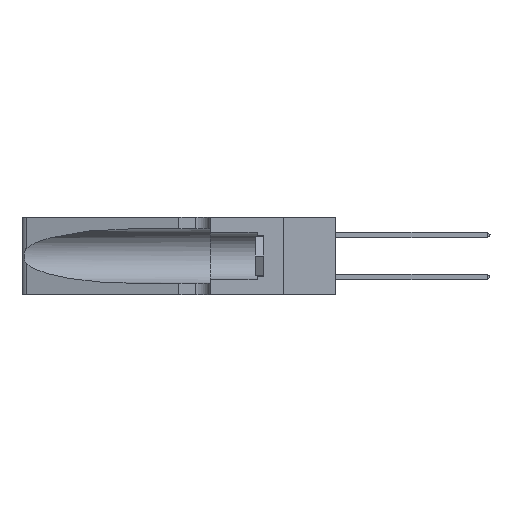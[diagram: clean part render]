
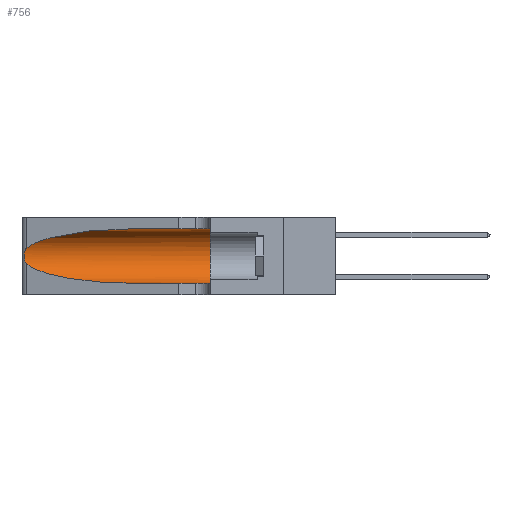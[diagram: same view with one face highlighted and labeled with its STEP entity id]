
A CAD part, left-side view. The second image highlights one B-rep face of the part: STEP entity #756.
In plain terms, the highlighted cylindrical face has radius 3.308 mm (diameter 6.617 mm), a partial arc.
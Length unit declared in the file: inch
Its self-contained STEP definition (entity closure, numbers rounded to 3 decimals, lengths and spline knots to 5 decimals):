
#478 = DIRECTION ( 'NONE',  ( 0., 1., 0. ) ) ;
#519 = CARTESIAN_POINT ( 'NONE',  ( 0.18966, 0.96281, 0.05475 ) ) ;
#756 = ADVANCED_FACE ( 'NONE', ( #10962 ), #19780, .F. ) ;
#801 = CARTESIAN_POINT ( 'NONE',  ( 0.1305, 0.35, 0.05475 ) ) ;
#1711 = CARTESIAN_POINT ( 'NONE',  ( 0.25639, 1.23186, 0.15144 ) ) ;
#2062 = CARTESIAN_POINT ( 'NONE',  ( 0.1305, 0.35, 0.31525 ) ) ;
#2937 = CARTESIAN_POINT ( 'NONE',  ( 0.25487, 1.22718, 0.22369 ) ) ;
#3628 = DIRECTION ( 'NONE',  ( 0., -1., 0. ) ) ;
#3702 = CARTESIAN_POINT ( 'NONE',  ( 0.25487, 1.22718, 0.14631 ) ) ;
#3805 = VECTOR ( 'NONE', #5480, 39.37008 ) ;
#3994 = VERTEX_POINT ( 'NONE', #6387 ) ;
#4312 = VERTEX_POINT ( 'NONE', #22398 ) ;
#4530 = VERTEX_POINT ( 'NONE', #24722 ) ;
#4669 = ORIENTED_EDGE ( 'NONE', *, *, #15088, .F. ) ;
#5480 = DIRECTION ( 'NONE',  ( 0., -1., 0. ) ) ;
#5661 = CARTESIAN_POINT ( 'NONE',  ( 0.25639, 1.23184, 0.21858 ) ) ;
#5757 =( BOUNDED_CURVE ( )  B_SPLINE_CURVE ( 3, ( #23375, #21598, #519, #14153 ),
 .UNSPECIFIED., .F., .F. ) 
 B_SPLINE_CURVE_WITH_KNOTS ( ( 4, 4 ),
 ( 3.44316, 4.71239 ),
 .UNSPECIFIED. ) 
 CURVE ( )  GEOMETRIC_REPRESENTATION_ITEM ( )  RATIONAL_B_SPLINE_CURVE ( ( 1., 0.87, 0.87, 1. ) ) 
 REPRESENTATION_ITEM ( '' )  );
#6387 = CARTESIAN_POINT ( 'NONE',  ( 0.1305, 0.72297, 0.31525 ) ) ;
#7619 = CARTESIAN_POINT ( 'NONE',  ( 0.25854, 1.2359, 0.20912 ) ) ;
#7921 = EDGE_CURVE ( 'NONE', #3994, #4530, #21419, .T. ) ;
#8882 = ORIENTED_EDGE ( 'NONE', *, *, #11031, .T. ) ;
#9578 = CARTESIAN_POINT ( 'NONE',  ( 0.26075, 1.23896, 0.19203 ) ) ;
#10030 = B_SPLINE_CURVE_WITH_KNOTS ( 'NONE', 3,
 ( #13295, #15187, #5661, #18964, #7619, #20837, #9578, #22679, #11482, #24537, #13374, #1711, #15270, #3702 ),
 .UNSPECIFIED., .F., .F.,
 ( 4, 2, 2, 2, 2, 2, 4 ),
 ( 0., 0.00027, 0.00053, 0.00107, 0.0016, 0.00187, 0.00214 ),
 .UNSPECIFIED. ) ;
#10962 = FACE_OUTER_BOUND ( 'NONE', #17174, .T. ) ;
#11031 = EDGE_CURVE ( 'NONE', #4530, #4312, #10030, .T. ) ;
#11482 = CARTESIAN_POINT ( 'NONE',  ( 0.26017, 1.23833, 0.17102 ) ) ;
#11982 = EDGE_CURVE ( 'NONE', #4312, #24225, #5757, .T. ) ;
#12139 = CARTESIAN_POINT ( 'NONE',  ( 0.1305, 1.61858, 0.185 ) ) ;
#12218 = CARTESIAN_POINT ( 'NONE',  ( 0.1305, 0.35, 0.185 ) ) ;
#12473 = ORIENTED_EDGE ( 'NONE', *, *, #11982, .T. ) ;
#12958 = DIRECTION ( 'NONE',  ( 0., -1., 0. ) ) ;
#13095 = VERTEX_POINT ( 'NONE', #2062 ) ;
#13295 = CARTESIAN_POINT ( 'NONE',  ( 0.25487, 1.22718, 0.22369 ) ) ;
#13374 = CARTESIAN_POINT ( 'NONE',  ( 0.25789, 1.23486, 0.15765 ) ) ;
#13762 = DIRECTION ( 'NONE',  ( 0., 0., -1. ) ) ;
#14127 = DIRECTION ( 'NONE',  ( 0., 0., 1. ) ) ;
#14153 = CARTESIAN_POINT ( 'NONE',  ( 0.1305, 0.72297, 0.05475 ) ) ;
#14269 = AXIS2_PLACEMENT_3D ( 'NONE', #12139, #12958, #13762 ) ;
#14525 = CARTESIAN_POINT ( 'NONE',  ( 0.2373, 1.15595, 0.28018 ) ) ;
#14857 = CARTESIAN_POINT ( 'NONE',  ( 0.1305, 0.72297, 0.05475 ) ) ;
#15036 = CARTESIAN_POINT ( 'NONE',  ( 0.1305, 1.61858, 0.31525 ) ) ;
#15088 = EDGE_CURVE ( 'NONE', #13095, #22888, #17392, .T. ) ;
#15187 = CARTESIAN_POINT ( 'NONE',  ( 0.25555, 1.22994, 0.2215 ) ) ;
#15270 = CARTESIAN_POINT ( 'NONE',  ( 0.25555, 1.22993, 0.14849 ) ) ;
#15970 = EDGE_CURVE ( 'NONE', #3994, #13095, #18520, .T. ) ;
#16364 = CARTESIAN_POINT ( 'NONE',  ( 0.18966, 0.96281, 0.31525 ) ) ;
#16573 = ORIENTED_EDGE ( 'NONE', *, *, #21259, .T. ) ;
#17174 = EDGE_LOOP ( 'NONE', ( #20546, #8882, #12473, #16573, #4669, #20761 ) ) ;
#17392 = CIRCLE ( 'NONE', #21376, 0.13025 ) ;
#18249 = CARTESIAN_POINT ( 'NONE',  ( 0.1305, 0.72297, 0.31525 ) ) ;
#18520 = LINE ( 'NONE', #15036, #3805 ) ;
#18964 = CARTESIAN_POINT ( 'NONE',  ( 0.25787, 1.23484, 0.2124 ) ) ;
#18978 = CARTESIAN_POINT ( 'NONE',  ( 0.1305, 1.61858, 0.05475 ) ) ;
#19780 = CYLINDRICAL_SURFACE ( 'NONE', #14269, 0.13025 ) ;
#19819 = LINE ( 'NONE', #18978, #24145 ) ;
#20546 = ORIENTED_EDGE ( 'NONE', *, *, #7921, .T. ) ;
#20761 = ORIENTED_EDGE ( 'NONE', *, *, #15970, .F. ) ;
#20837 = CARTESIAN_POINT ( 'NONE',  ( 0.26018, 1.23835, 0.19895 ) ) ;
#21259 = EDGE_CURVE ( 'NONE', #24225, #22888, #19819, .T. ) ;
#21376 = AXIS2_PLACEMENT_3D ( 'NONE', #12218, #478, #14127 ) ;
#21419 =( BOUNDED_CURVE ( )  B_SPLINE_CURVE ( 3, ( #18249, #16364, #14525, #2937 ),
 .UNSPECIFIED., .F., .F. ) 
 B_SPLINE_CURVE_WITH_KNOTS ( ( 4, 4 ),
 ( 1.5708, 2.84003 ),
 .UNSPECIFIED. ) 
 CURVE ( )  GEOMETRIC_REPRESENTATION_ITEM ( )  RATIONAL_B_SPLINE_CURVE ( ( 1., 0.87, 0.87, 1. ) ) 
 REPRESENTATION_ITEM ( '' )  );
#21598 = CARTESIAN_POINT ( 'NONE',  ( 0.2373, 1.15595, 0.08982 ) ) ;
#22398 = CARTESIAN_POINT ( 'NONE',  ( 0.25487, 1.22718, 0.14631 ) ) ;
#22679 = CARTESIAN_POINT ( 'NONE',  ( 0.26075, 1.23896, 0.178 ) ) ;
#22888 = VERTEX_POINT ( 'NONE', #801 ) ;
#23375 = CARTESIAN_POINT ( 'NONE',  ( 0.25487, 1.22718, 0.14631 ) ) ;
#24145 = VECTOR ( 'NONE', #3628, 39.37008 ) ;
#24225 = VERTEX_POINT ( 'NONE', #14857 ) ;
#24537 = CARTESIAN_POINT ( 'NONE',  ( 0.25856, 1.23593, 0.16098 ) ) ;
#24722 = CARTESIAN_POINT ( 'NONE',  ( 0.25487, 1.22718, 0.22369 ) ) ;
